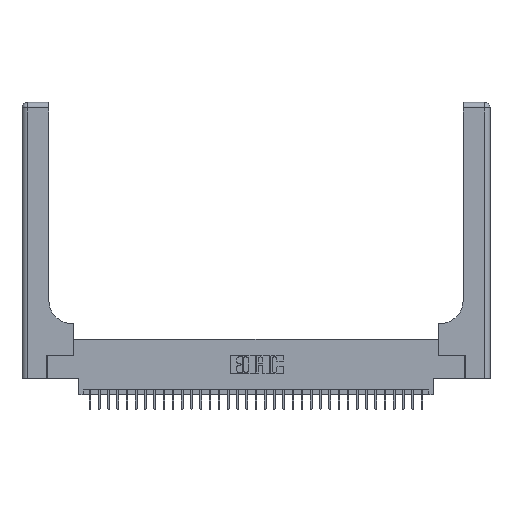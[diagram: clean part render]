
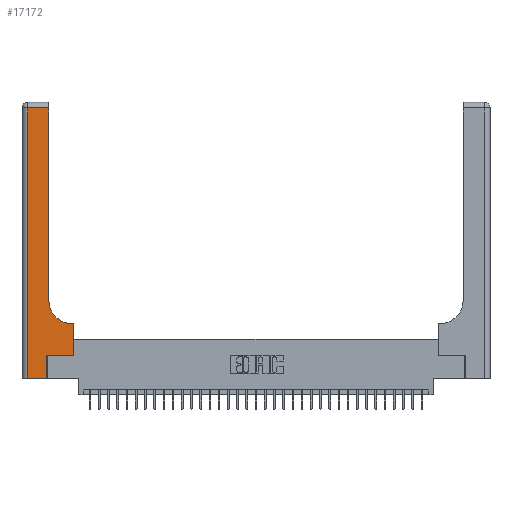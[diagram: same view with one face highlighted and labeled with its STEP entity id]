
A CAD part, top view. The second image highlights one B-rep face of the part: STEP entity #17172.
In plain terms, the highlighted planar face has unit normal (0, 0, 1).
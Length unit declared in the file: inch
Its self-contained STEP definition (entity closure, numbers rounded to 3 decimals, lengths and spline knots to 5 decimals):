
#331 = LINE ( 'NONE', #29671, #23249 ) ;
#1220 = EDGE_CURVE ( 'NONE', #29876, #14805, #29882, .T. ) ;
#1245 = CARTESIAN_POINT ( 'NONE',  ( 0.5585, 0.25, 0.37 ) ) ;
#1725 = DIRECTION ( 'NONE',  ( 1., 0., 0. ) ) ;
#2152 = CARTESIAN_POINT ( 'NONE',  ( 0.2915, 3., 0.37 ) ) ;
#2200 = DIRECTION ( 'NONE',  ( 0., 0., -1. ) ) ;
#3086 = CARTESIAN_POINT ( 'NONE',  ( 0.06, 2.94, 0.37 ) ) ;
#3402 = CARTESIAN_POINT ( 'NONE',  ( 0.269, 0.25, 0.37 ) ) ;
#4134 = CARTESIAN_POINT ( 'NONE',  ( 0.269, 0., 0.37 ) ) ;
#4570 = EDGE_CURVE ( 'NONE', #13916, #11228, #331, .T. ) ;
#4586 = CARTESIAN_POINT ( 'NONE',  ( 0.5415, 0.85, 0.37 ) ) ;
#4994 = DIRECTION ( 'NONE',  ( -1., 0., 0. ) ) ;
#5234 = VERTEX_POINT ( 'NONE', #14788 ) ;
#5268 = VECTOR ( 'NONE', #23728, 39.37008 ) ;
#5310 = VERTEX_POINT ( 'NONE', #3402 ) ;
#5483 = ORIENTED_EDGE ( 'NONE', *, *, #16328, .T. ) ;
#6812 = ORIENTED_EDGE ( 'NONE', *, *, #17078, .T. ) ;
#7495 = LINE ( 'NONE', #17757, #23962 ) ;
#7717 = ORIENTED_EDGE ( 'NONE', *, *, #27618, .T. ) ;
#8008 = CARTESIAN_POINT ( 'NONE',  ( 0., 2.94, 0.37 ) ) ;
#8137 = DIRECTION ( 'NONE',  ( 1., 0., 0. ) ) ;
#9020 = DIRECTION ( 'NONE',  ( -1., 0., 0. ) ) ;
#9760 = DIRECTION ( 'NONE',  ( 1., 0., 0. ) ) ;
#10836 = EDGE_CURVE ( 'NONE', #16870, #29366, #11327, .T. ) ;
#11144 = VECTOR ( 'NONE', #34113, 39.37008 ) ;
#11228 = VERTEX_POINT ( 'NONE', #4134 ) ;
#11327 = LINE ( 'NONE', #8008, #32246 ) ;
#11967 = EDGE_LOOP ( 'NONE', ( #18658, #13144, #7717, #17589, #29201, #5483, #24863, #6812, #21702 ) ) ;
#12285 = LINE ( 'NONE', #34878, #27143 ) ;
#12715 = VERTEX_POINT ( 'NONE', #17186 ) ;
#13133 = LINE ( 'NONE', #18209, #19435 ) ;
#13144 = ORIENTED_EDGE ( 'NONE', *, *, #10836, .T. ) ;
#13916 = VERTEX_POINT ( 'NONE', #28247 ) ;
#14788 = CARTESIAN_POINT ( 'NONE',  ( 0.5585, 0.25, 0.37 ) ) ;
#14805 = VERTEX_POINT ( 'NONE', #26018 ) ;
#15396 = DIRECTION ( 'NONE',  ( 0., -1., 0. ) ) ;
#16328 = EDGE_CURVE ( 'NONE', #5310, #5234, #13133, .T. ) ;
#16870 = VERTEX_POINT ( 'NONE', #22718 ) ;
#17065 = DIRECTION ( 'NONE',  ( 0., 1., 0. ) ) ;
#17078 = EDGE_CURVE ( 'NONE', #12715, #29876, #12285, .T. ) ;
#17172 = ADVANCED_FACE ( 'NONE', ( #31730 ), #35109, .F. ) ;
#17186 = CARTESIAN_POINT ( 'NONE',  ( 0.5585, 0.6, 0.37 ) ) ;
#17589 = ORIENTED_EDGE ( 'NONE', *, *, #4570, .T. ) ;
#17757 = CARTESIAN_POINT ( 'NONE',  ( 0.06, 3., 0.37 ) ) ;
#18209 = CARTESIAN_POINT ( 'NONE',  ( 0.269, 0.25, 0.37 ) ) ;
#18315 = CARTESIAN_POINT ( 'NONE',  ( 0., 3., 0.37 ) ) ;
#18404 = EDGE_CURVE ( 'NONE', #5234, #12715, #20046, .T. ) ;
#18641 = AXIS2_PLACEMENT_3D ( 'NONE', #18315, #2200, #4994 ) ;
#18658 = ORIENTED_EDGE ( 'NONE', *, *, #19004, .T. ) ;
#19004 = EDGE_CURVE ( 'NONE', #14805, #16870, #20052, .T. ) ;
#19435 = VECTOR ( 'NONE', #1725, 39.37008 ) ;
#19848 = AXIS2_PLACEMENT_3D ( 'NONE', #4586, #34592, #9760 ) ;
#20046 = LINE ( 'NONE', #1245, #11144 ) ;
#20052 = LINE ( 'NONE', #2152, #5268 ) ;
#20981 = LINE ( 'NONE', #28402, #22632 ) ;
#21702 = ORIENTED_EDGE ( 'NONE', *, *, #1220, .T. ) ;
#22632 = VECTOR ( 'NONE', #17065, 39.37008 ) ;
#22718 = CARTESIAN_POINT ( 'NONE',  ( 0.2915, 2.94, 0.37 ) ) ;
#23249 = VECTOR ( 'NONE', #8137, 39.37008 ) ;
#23728 = DIRECTION ( 'NONE',  ( 0., 1., 0. ) ) ;
#23962 = VECTOR ( 'NONE', #15396, 39.37008 ) ;
#24235 = DIRECTION ( 'NONE',  ( -1., 0., 0. ) ) ;
#24863 = ORIENTED_EDGE ( 'NONE', *, *, #18404, .T. ) ;
#26018 = CARTESIAN_POINT ( 'NONE',  ( 0.2915, 0.85, 0.37 ) ) ;
#27143 = VECTOR ( 'NONE', #24235, 39.37008 ) ;
#27618 = EDGE_CURVE ( 'NONE', #29366, #13916, #7495, .T. ) ;
#27933 = EDGE_CURVE ( 'NONE', #11228, #5310, #20981, .T. ) ;
#28247 = CARTESIAN_POINT ( 'NONE',  ( 0.06, 0., 0.37 ) ) ;
#28402 = CARTESIAN_POINT ( 'NONE',  ( 0.269, 0., 0.37 ) ) ;
#29075 = CARTESIAN_POINT ( 'NONE',  ( 0.5415, 0.6, 0.37 ) ) ;
#29201 = ORIENTED_EDGE ( 'NONE', *, *, #27933, .T. ) ;
#29366 = VERTEX_POINT ( 'NONE', #3086 ) ;
#29671 = CARTESIAN_POINT ( 'NONE',  ( 0., 0., 0.37 ) ) ;
#29876 = VERTEX_POINT ( 'NONE', #29075 ) ;
#29882 = CIRCLE ( 'NONE', #19848, 0.25 ) ;
#31730 = FACE_OUTER_BOUND ( 'NONE', #11967, .T. ) ;
#32246 = VECTOR ( 'NONE', #9020, 39.37008 ) ;
#34113 = DIRECTION ( 'NONE',  ( 0., 1., 0. ) ) ;
#34592 = DIRECTION ( 'NONE',  ( 0., 0., -1. ) ) ;
#34878 = CARTESIAN_POINT ( 'NONE',  ( 0.2915, 0.6, 0.37 ) ) ;
#35109 = PLANE ( 'NONE',  #18641 ) ;
